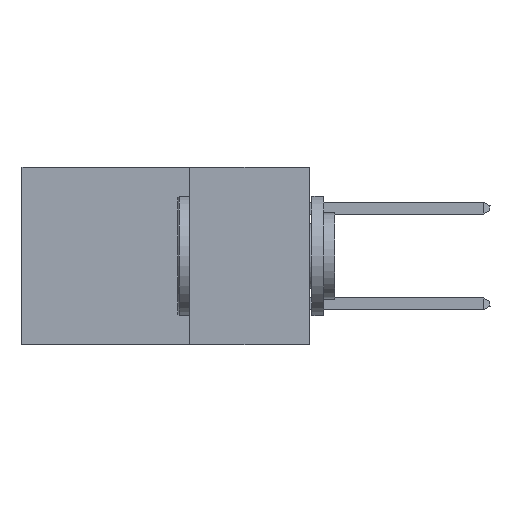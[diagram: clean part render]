
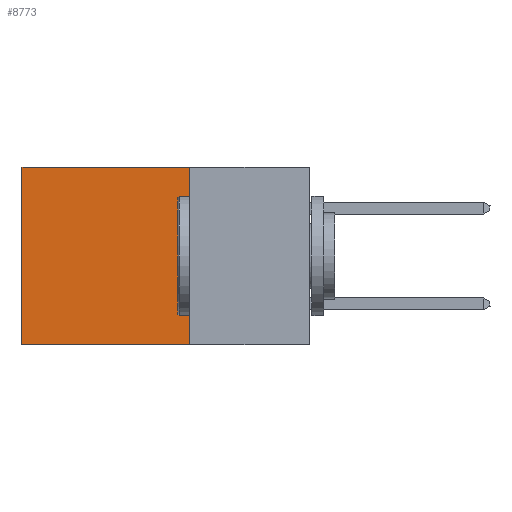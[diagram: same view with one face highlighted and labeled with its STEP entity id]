
A CAD part, left-side view. The second image highlights one B-rep face of the part: STEP entity #8773.
In plain terms, the highlighted planar face has unit normal (-1, 0, 0).
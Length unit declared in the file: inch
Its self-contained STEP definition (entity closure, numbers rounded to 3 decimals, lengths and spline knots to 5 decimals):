
#341 = LINE ( 'NONE', #6954, #7561 ) ;
#472 = CARTESIAN_POINT ( 'NONE',  ( 0.2875, 0.25, 0. ) ) ;
#624 = CARTESIAN_POINT ( 'NONE',  ( 0.2875, 0.6, 0. ) ) ;
#960 = ORIENTED_EDGE ( 'NONE', *, *, #16289, .T. ) ;
#1058 = PLANE ( 'NONE',  #8623 ) ;
#1106 = CARTESIAN_POINT ( 'NONE',  ( 0.2875, 0.25, 0. ) ) ;
#1169 = DIRECTION ( 'NONE',  ( 0., 0., -1. ) ) ;
#2467 = CARTESIAN_POINT ( 'NONE',  ( 0.2875, 0.25, 0. ) ) ;
#2571 = DIRECTION ( 'NONE',  ( 0., 0., -1. ) ) ;
#2771 = LINE ( 'NONE', #1106, #12494 ) ;
#4234 = CARTESIAN_POINT ( 'NONE',  ( 0.2875, 0.6, 0. ) ) ;
#4676 = CARTESIAN_POINT ( 'NONE',  ( 0.2875, 0.6, -0.37 ) ) ;
#4926 = LINE ( 'NONE', #16615, #5367 ) ;
#5198 = ORIENTED_EDGE ( 'NONE', *, *, #16294, .F. ) ;
#5367 = VECTOR ( 'NONE', #18390, 39.37008 ) ;
#6954 = CARTESIAN_POINT ( 'NONE',  ( 0.2875, 0.25, 0. ) ) ;
#7058 = LINE ( 'NONE', #4234, #15850 ) ;
#7561 = VECTOR ( 'NONE', #2571, 39.37008 ) ;
#8623 = AXIS2_PLACEMENT_3D ( 'NONE', #2467, #16962, #16734 ) ;
#8670 = VERTEX_POINT ( 'NONE', #624 ) ;
#8773 = ADVANCED_FACE ( 'NONE', ( #16177 ), #1058, .F. ) ;
#9487 = ORIENTED_EDGE ( 'NONE', *, *, #11201, .T. ) ;
#10598 = VERTEX_POINT ( 'NONE', #17369 ) ;
#11201 = EDGE_CURVE ( 'NONE', #8670, #11450, #7058, .T. ) ;
#11450 = VERTEX_POINT ( 'NONE', #4676 ) ;
#12494 = VECTOR ( 'NONE', #17204, 39.37008 ) ;
#14254 = VERTEX_POINT ( 'NONE', #472 ) ;
#15850 = VECTOR ( 'NONE', #1169, 39.37008 ) ;
#16177 = FACE_OUTER_BOUND ( 'NONE', #17362, .T. ) ;
#16289 = EDGE_CURVE ( 'NONE', #14254, #8670, #2771, .T. ) ;
#16294 = EDGE_CURVE ( 'NONE', #14254, #10598, #341, .T. ) ;
#16615 = CARTESIAN_POINT ( 'NONE',  ( 0.2875, 0.25, -0.37 ) ) ;
#16734 = DIRECTION ( 'NONE',  ( 0., 0., -1. ) ) ;
#16962 = DIRECTION ( 'NONE',  ( 1., 0., 0. ) ) ;
#17167 = ORIENTED_EDGE ( 'NONE', *, *, #17438, .F. ) ;
#17204 = DIRECTION ( 'NONE',  ( 0., 1., 0. ) ) ;
#17362 = EDGE_LOOP ( 'NONE', ( #9487, #17167, #5198, #960 ) ) ;
#17369 = CARTESIAN_POINT ( 'NONE',  ( 0.2875, 0.25, -0.37 ) ) ;
#17438 = EDGE_CURVE ( 'NONE', #10598, #11450, #4926, .T. ) ;
#18390 = DIRECTION ( 'NONE',  ( 0., 1., 0. ) ) ;
